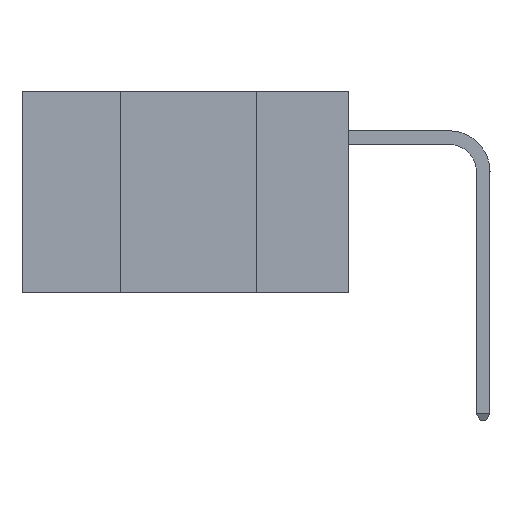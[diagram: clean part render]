
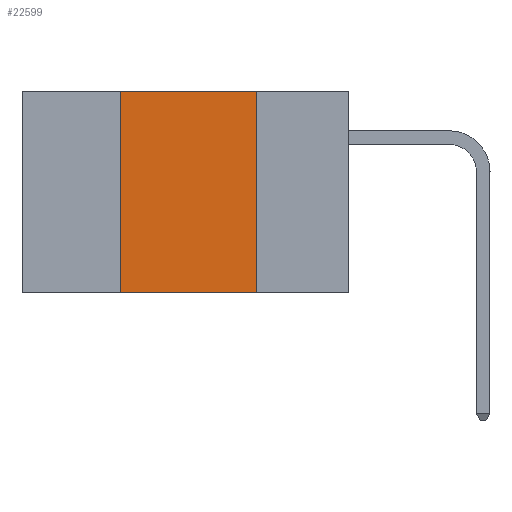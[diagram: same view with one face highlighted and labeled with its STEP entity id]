
A CAD part, left-side view. The second image highlights one B-rep face of the part: STEP entity #22599.
In plain terms, the highlighted planar face has unit normal (-1, 0, 0).
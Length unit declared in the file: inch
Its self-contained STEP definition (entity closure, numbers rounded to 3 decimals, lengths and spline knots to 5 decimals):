
#1356 = EDGE_CURVE ( 'NONE', #23097, #6528, #18967, .T. ) ;
#2171 = CARTESIAN_POINT ( 'NONE',  ( 0., 0.6, -0.37 ) ) ;
#3135 = CARTESIAN_POINT ( 'NONE',  ( 0., 0.17, 0. ) ) ;
#3581 = CARTESIAN_POINT ( 'NONE',  ( 0., 0.17, 0. ) ) ;
#5473 = EDGE_LOOP ( 'NONE', ( #25381, #18099, #32138, #8733 ) ) ;
#5932 = DIRECTION ( 'NONE',  ( 0., 0., 1. ) ) ;
#6528 = VERTEX_POINT ( 'NONE', #12002 ) ;
#7269 = EDGE_CURVE ( 'NONE', #24079, #6528, #28830, .T. ) ;
#7281 = VECTOR ( 'NONE', #5932, 39.37008 ) ;
#7446 = PLANE ( 'NONE',  #7660 ) ;
#7660 = AXIS2_PLACEMENT_3D ( 'NONE', #9939, #29966, #14986 ) ;
#8688 = DIRECTION ( 'NONE',  ( 0., -1., 0. ) ) ;
#8733 = ORIENTED_EDGE ( 'NONE', *, *, #1356, .T. ) ;
#8874 = VECTOR ( 'NONE', #18531, 39.37008 ) ;
#9939 = CARTESIAN_POINT ( 'NONE',  ( 0., 0.6, 0. ) ) ;
#12002 = CARTESIAN_POINT ( 'NONE',  ( 0., 0.17, -0.37 ) ) ;
#13568 = CARTESIAN_POINT ( 'NONE',  ( 0., 0.42, 0. ) ) ;
#13693 = LINE ( 'NONE', #23795, #26233 ) ;
#13931 = LINE ( 'NONE', #30847, #7281 ) ;
#14986 = DIRECTION ( 'NONE',  ( 0., 0., -1. ) ) ;
#18099 = ORIENTED_EDGE ( 'NONE', *, *, #26161, .F. ) ;
#18531 = DIRECTION ( 'NONE',  ( 0., 0., -1. ) ) ;
#18967 = LINE ( 'NONE', #2171, #24499 ) ;
#21332 = EDGE_CURVE ( 'NONE', #23097, #24177, #13931, .T. ) ;
#22599 = ADVANCED_FACE ( 'NONE', ( #23751 ), #7446, .F. ) ;
#23097 = VERTEX_POINT ( 'NONE', #26781 ) ;
#23751 = FACE_OUTER_BOUND ( 'NONE', #5473, .T. ) ;
#23795 = CARTESIAN_POINT ( 'NONE',  ( 0., 0.6, 0. ) ) ;
#24079 = VERTEX_POINT ( 'NONE', #3135 ) ;
#24177 = VERTEX_POINT ( 'NONE', #13568 ) ;
#24499 = VECTOR ( 'NONE', #27165, 39.37008 ) ;
#25381 = ORIENTED_EDGE ( 'NONE', *, *, #7269, .F. ) ;
#26161 = EDGE_CURVE ( 'NONE', #24177, #24079, #13693, .T. ) ;
#26233 = VECTOR ( 'NONE', #8688, 39.37008 ) ;
#26781 = CARTESIAN_POINT ( 'NONE',  ( 0., 0.42, -0.37 ) ) ;
#27165 = DIRECTION ( 'NONE',  ( 0., -1., 0. ) ) ;
#28830 = LINE ( 'NONE', #3581, #8874 ) ;
#29966 = DIRECTION ( 'NONE',  ( 1., 0., 0. ) ) ;
#30847 = CARTESIAN_POINT ( 'NONE',  ( 0., 0.42, 0. ) ) ;
#32138 = ORIENTED_EDGE ( 'NONE', *, *, #21332, .F. ) ;
